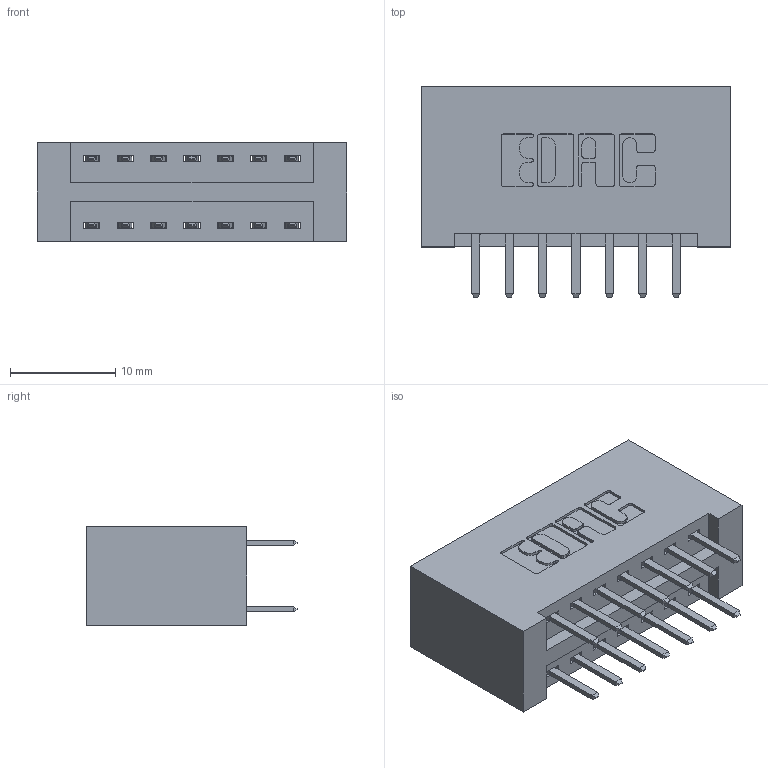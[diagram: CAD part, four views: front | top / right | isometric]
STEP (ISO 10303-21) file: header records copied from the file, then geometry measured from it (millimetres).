
FILE_DESCRIPTION (( 'STEP AP203' ), '1' );
FILE_NAME ('396-014-520-201.STEP', '2019-10-29T19:47:15', ( '' ), ( '' ), 'SwSTEP 2.0', 'SolidWorks 2016', '' );
FILE_SCHEMA (( 'CONFIG_CONTROL_DESIGN' ));
Length unit declared in the file: inch
Products named in the file (3): 345-292-001_345-293-120; 346 Part_No Mounting Lugs; 396-014-520-201
Assembly tree (15 placements, depth 2):
  396-014-520-201
    346 Part_No Mounting Lugs
    345-292-001_345-293-120  x14
Bounding box: 29.46 x 20.02 x 9.4 mm (x, y, z)
Volume: 3168.4 mm3; surface area: 3953.8 mm2
Topology: 15 solids, 15 shells, 898 faces, 2587 edges, 1686 vertices
Faces by surface type: plane 590, cylinder 308
Entity records: 9117 total; most frequent: CARTESIAN_POINT 1560, ORIENTED_EDGE 1482, DIRECTION 1409, EDGE_CURVE 741, VECTOR 585, LINE 585, VERTEX_POINT 490, AXIS2_PLACEMENT_3D 412
